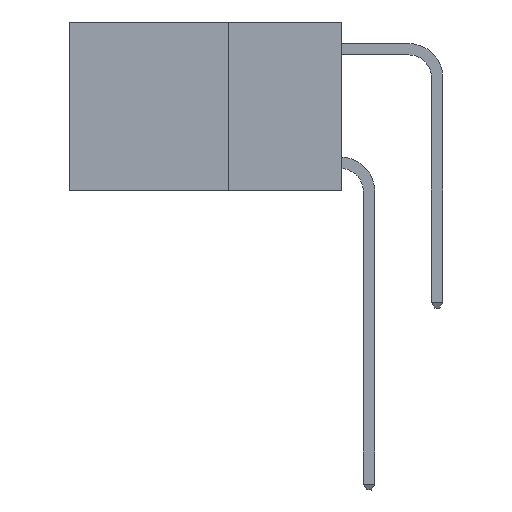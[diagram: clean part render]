
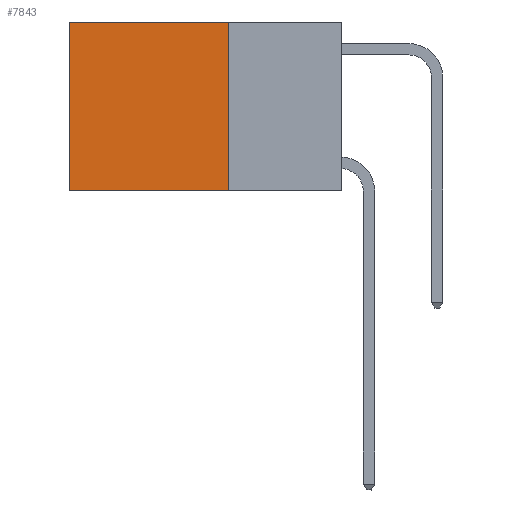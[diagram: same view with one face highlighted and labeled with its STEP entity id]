
A CAD part, left-side view. The second image highlights one B-rep face of the part: STEP entity #7843.
In plain terms, the highlighted planar face has unit normal (-1, 0, 0).
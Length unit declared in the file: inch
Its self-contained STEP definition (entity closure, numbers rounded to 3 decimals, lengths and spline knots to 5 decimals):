
#328 = CARTESIAN_POINT ( 'NONE',  ( 0.2625, 0.6, -0.37 ) ) ;
#1392 = CARTESIAN_POINT ( 'NONE',  ( 0.2625, 0.25, -0.37 ) ) ;
#1667 = CARTESIAN_POINT ( 'NONE',  ( 0.2625, 0.25, -0.37 ) ) ;
#2301 = DIRECTION ( 'NONE',  ( 0., 1., 0. ) ) ;
#2478 = CARTESIAN_POINT ( 'NONE',  ( 0.2625, 0.25, 0. ) ) ;
#2659 = EDGE_CURVE ( 'NONE', #2751, #4391, #4458, .T. ) ;
#2751 = VERTEX_POINT ( 'NONE', #6073 ) ;
#2789 = VERTEX_POINT ( 'NONE', #7956 ) ;
#2801 = DIRECTION ( 'NONE',  ( 0., 0., -1. ) ) ;
#3084 = DIRECTION ( 'NONE',  ( 0., 0., -1. ) ) ;
#3472 = VECTOR ( 'NONE', #2301, 39.37008 ) ;
#3756 = ORIENTED_EDGE ( 'NONE', *, *, #7513, .T. ) ;
#3767 = ORIENTED_EDGE ( 'NONE', *, *, #2659, .F. ) ;
#3801 = LINE ( 'NONE', #10053, #7995 ) ;
#3903 = ORIENTED_EDGE ( 'NONE', *, *, #4121, .F. ) ;
#4004 = ORIENTED_EDGE ( 'NONE', *, *, #8299, .T. ) ;
#4121 = EDGE_CURVE ( 'NONE', #4391, #7919, #5802, .T. ) ;
#4391 = VERTEX_POINT ( 'NONE', #1667 ) ;
#4458 = LINE ( 'NONE', #2478, #7365 ) ;
#5384 = CARTESIAN_POINT ( 'NONE',  ( 0.2625, 0.25, 0. ) ) ;
#5802 = LINE ( 'NONE', #1392, #3472 ) ;
#6073 = CARTESIAN_POINT ( 'NONE',  ( 0.2625, 0.25, 0. ) ) ;
#7072 = FACE_OUTER_BOUND ( 'NONE', #8388, .T. ) ;
#7165 = PLANE ( 'NONE',  #9766 ) ;
#7365 = VECTOR ( 'NONE', #7787, 39.37008 ) ;
#7513 = EDGE_CURVE ( 'NONE', #2751, #2789, #3801, .T. ) ;
#7787 = DIRECTION ( 'NONE',  ( 0., 0., -1. ) ) ;
#7843 = ADVANCED_FACE ( 'NONE', ( #7072 ), #7165, .F. ) ;
#7919 = VERTEX_POINT ( 'NONE', #328 ) ;
#7956 = CARTESIAN_POINT ( 'NONE',  ( 0.2625, 0.6, 0. ) ) ;
#7995 = VECTOR ( 'NONE', #8194, 39.37008 ) ;
#8135 = DIRECTION ( 'NONE',  ( 1., 0., 0. ) ) ;
#8194 = DIRECTION ( 'NONE',  ( 0., 1., 0. ) ) ;
#8256 = LINE ( 'NONE', #8458, #10728 ) ;
#8299 = EDGE_CURVE ( 'NONE', #2789, #7919, #8256, .T. ) ;
#8388 = EDGE_LOOP ( 'NONE', ( #4004, #3903, #3767, #3756 ) ) ;
#8458 = CARTESIAN_POINT ( 'NONE',  ( 0.2625, 0.6, 0. ) ) ;
#9766 = AXIS2_PLACEMENT_3D ( 'NONE', #5384, #8135, #2801 ) ;
#10053 = CARTESIAN_POINT ( 'NONE',  ( 0.2625, 0.25, 0. ) ) ;
#10728 = VECTOR ( 'NONE', #3084, 39.37008 ) ;
